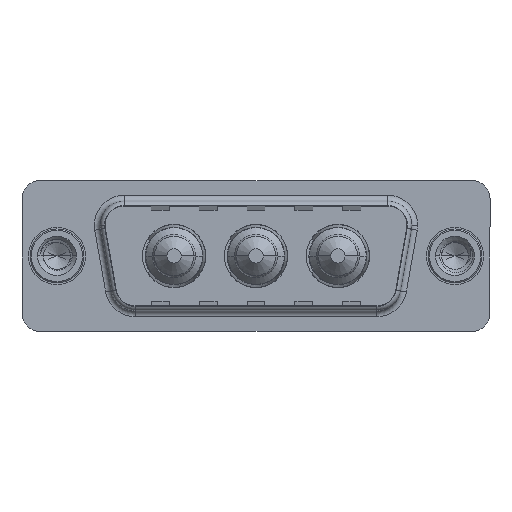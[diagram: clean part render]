
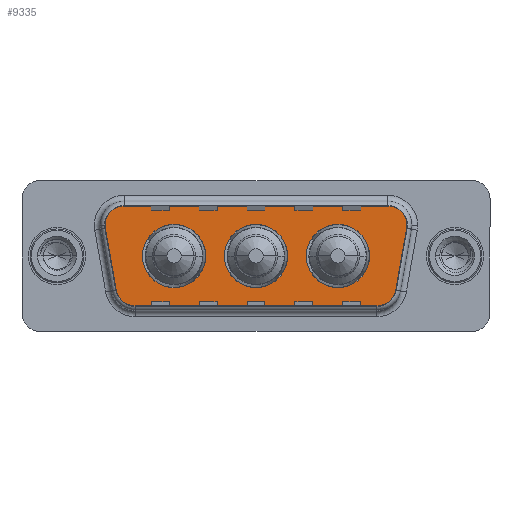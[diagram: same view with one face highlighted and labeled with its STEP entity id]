
A CAD part, top view. The second image highlights one B-rep face of the part: STEP entity #9335.
In plain terms, the highlighted planar face has unit normal (0, 0, 1).
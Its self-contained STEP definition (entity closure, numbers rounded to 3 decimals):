
#252 = CARTESIAN_POINT ( 'NONE',  ( 5.411, 4.9, 0. ) ) ;
#333 = DIRECTION ( 'NONE',  ( -1., 0., 0. ) ) ;
#359 = FACE_BOUND ( 'NONE', #11732, .T. ) ;
#482 = CARTESIAN_POINT ( 'NONE',  ( 14., 0., 0. ) ) ;
#794 = CARTESIAN_POINT ( 'NONE',  ( 29.859, 2.553, 0. ) ) ;
#1148 = VECTOR ( 'NONE', #8163, 1000. ) ;
#1615 = CIRCLE ( 'NONE', #15062, 2.65 ) ;
#1668 = EDGE_LOOP ( 'NONE', ( #4404, #13448 ) ) ;
#1833 = AXIS2_PLACEMENT_3D ( 'NONE', #14568, #5137, #16014 ) ;
#2501 = DIRECTION ( 'NONE',  ( 1., 0., 0. ) ) ;
#2558 = CARTESIAN_POINT ( 'NONE',  ( 16.65, 0., 0. ) ) ;
#2689 = DIRECTION ( 'NONE',  ( 0., 0., 1. ) ) ;
#2873 = VERTEX_POINT ( 'NONE', #482 ) ;
#3039 = CARTESIAN_POINT ( 'NONE',  ( 6.434, -4.9, 0. ) ) ;
#3252 = CARTESIAN_POINT ( 'NONE',  ( 12.45, 0., 0. ) ) ;
#3286 = VERTEX_POINT ( 'NONE', #19120 ) ;
#3309 = EDGE_CURVE ( 'NONE', #6683, #13294, #7062, .T. ) ;
#3829 = AXIS2_PLACEMENT_3D ( 'NONE', #7173, #17907, #8789 ) ;
#3975 = FACE_BOUND ( 'NONE', #1668, .T. ) ;
#3980 = CARTESIAN_POINT ( 'NONE',  ( 26.866, -2.9, 0. ) ) ;
#4006 = CARTESIAN_POINT ( 'NONE',  ( 6.434, -4.9, 0. ) ) ;
#4015 = DIRECTION ( 'NONE',  ( 0., 0., 1. ) ) ;
#4022 = CARTESIAN_POINT ( 'NONE',  ( 27.889, 2.9, 0. ) ) ;
#4078 = EDGE_CURVE ( 'NONE', #5817, #15979, #13440, .T. ) ;
#4096 = DIRECTION ( 'NONE',  ( 1., 0., 0. ) ) ;
#4179 = VERTEX_POINT ( 'NONE', #252 ) ;
#4404 = ORIENTED_EDGE ( 'NONE', *, *, #16567, .F. ) ;
#4530 = ORIENTED_EDGE ( 'NONE', *, *, #15115, .T. ) ;
#4539 = CARTESIAN_POINT ( 'NONE',  ( 7.15, 0., 0. ) ) ;
#4577 = CARTESIAN_POINT ( 'NONE',  ( 9.8, 0., 0. ) ) ;
#4589 = DIRECTION ( 'NONE',  ( 0., 0., 1. ) ) ;
#4745 = VECTOR ( 'NONE', #19899, 1000. ) ;
#4818 = VERTEX_POINT ( 'NONE', #15061 ) ;
#4990 = CARTESIAN_POINT ( 'NONE',  ( 5.411, 2.9, 0. ) ) ;
#5137 = DIRECTION ( 'NONE',  ( 0., 0., 1. ) ) ;
#5651 = ORIENTED_EDGE ( 'NONE', *, *, #4078, .F. ) ;
#5777 = LINE ( 'NONE', #11370, #1148 ) ;
#5817 = VERTEX_POINT ( 'NONE', #3252 ) ;
#5860 = AXIS2_PLACEMENT_3D ( 'NONE', #3980, #11973, #2501 ) ;
#5919 = EDGE_CURVE ( 'NONE', #16298, #8431, #14353, .T. ) ;
#6026 = VECTOR ( 'NONE', #16342, 1000. ) ;
#6195 = DIRECTION ( 'NONE',  ( 1., 0., 0. ) ) ;
#6215 = EDGE_CURVE ( 'NONE', #19218, #4818, #6723, .T. ) ;
#6226 = CARTESIAN_POINT ( 'NONE',  ( 26.15, 0., 0. ) ) ;
#6251 = CARTESIAN_POINT ( 'NONE',  ( 23.5, 0., 0. ) ) ;
#6263 = VERTEX_POINT ( 'NONE', #17975 ) ;
#6264 = EDGE_CURVE ( 'NONE', #2873, #7262, #17558, .T. ) ;
#6441 = DIRECTION ( 'NONE',  ( 1., 0., 0. ) ) ;
#6628 = DIRECTION ( 'NONE',  ( 1., 0., 0. ) ) ;
#6683 = VERTEX_POINT ( 'NONE', #19799 ) ;
#6723 = CIRCLE ( 'NONE', #3829, 2.65 ) ;
#6942 = DIRECTION ( 'NONE',  ( 0., 0., 1. ) ) ;
#6947 = CARTESIAN_POINT ( 'NONE',  ( 9.8, 0., 0. ) ) ;
#7012 = DIRECTION ( 'NONE',  ( 0.174, 0.985, 0. ) ) ;
#7062 = CIRCLE ( 'NONE', #19396, 2. ) ;
#7173 = CARTESIAN_POINT ( 'NONE',  ( 23.5, 0., 0. ) ) ;
#7262 = VERTEX_POINT ( 'NONE', #16443 ) ;
#7380 = CARTESIAN_POINT ( 'NONE',  ( 29.859, 2.553, 0. ) ) ;
#7455 = EDGE_CURVE ( 'NONE', #15979, #5817, #15241, .T. ) ;
#7823 = VERTEX_POINT ( 'NONE', #18087 ) ;
#7849 = DIRECTION ( 'NONE',  ( 1., 0., 0. ) ) ;
#7920 = AXIS2_PLACEMENT_3D ( 'NONE', #12153, #2689, #13696 ) ;
#8163 = DIRECTION ( 'NONE',  ( -1., 0., 0. ) ) ;
#8219 = FACE_BOUND ( 'NONE', #15372, .T. ) ;
#8285 = ORIENTED_EDGE ( 'NONE', *, *, #14871, .T. ) ;
#8373 = ORIENTED_EDGE ( 'NONE', *, *, #6215, .F. ) ;
#8431 = VERTEX_POINT ( 'NONE', #4006 ) ;
#8505 = AXIS2_PLACEMENT_3D ( 'NONE', #18816, #9777, #333 ) ;
#8544 = CIRCLE ( 'NONE', #1833, 2. ) ;
#8555 = ORIENTED_EDGE ( 'NONE', *, *, #10106, .T. ) ;
#8789 = DIRECTION ( 'NONE',  ( 1., 0., 0. ) ) ;
#8820 = ORIENTED_EDGE ( 'NONE', *, *, #7455, .F. ) ;
#9335 = ADVANCED_FACE ( 'NONE', ( #3975, #8219, #359, #19832 ), #10388, .T. ) ;
#9551 = ORIENTED_EDGE ( 'NONE', *, *, #17313, .T. ) ;
#9777 = DIRECTION ( 'NONE',  ( 0., 0., 1. ) ) ;
#9946 = VECTOR ( 'NONE', #7012, 1000. ) ;
#9954 = AXIS2_PLACEMENT_3D ( 'NONE', #4990, #15885, #6628 ) ;
#10106 = EDGE_CURVE ( 'NONE', #3286, #19796, #14539, .T. ) ;
#10279 = LINE ( 'NONE', #14810, #6026 ) ;
#10388 = PLANE ( 'NONE',  #5860 ) ;
#10881 = AXIS2_PLACEMENT_3D ( 'NONE', #14055, #4589, #15518 ) ;
#11247 = CIRCLE ( 'NONE', #9954, 2. ) ;
#11281 = AXIS2_PLACEMENT_3D ( 'NONE', #6947, #6942, #6441 ) ;
#11370 = CARTESIAN_POINT ( 'NONE',  ( 5.411, 4.9, 0. ) ) ;
#11732 = EDGE_LOOP ( 'NONE', ( #5651, #8820 ) ) ;
#11973 = DIRECTION ( 'NONE',  ( 0., 0., 1. ) ) ;
#12153 = CARTESIAN_POINT ( 'NONE',  ( 16.65, 0., 0. ) ) ;
#12320 = AXIS2_PLACEMENT_3D ( 'NONE', #2558, #13556, #4096 ) ;
#12523 = EDGE_LOOP ( 'NONE', ( #14360, #8555, #16471, #17594, #8285, #17183, #4530, #17198, #9551 ) ) ;
#12856 = AXIS2_PLACEMENT_3D ( 'NONE', #4577, #15508, #6195 ) ;
#13294 = VERTEX_POINT ( 'NONE', #15830 ) ;
#13440 = CIRCLE ( 'NONE', #11281, 2.65 ) ;
#13448 = ORIENTED_EDGE ( 'NONE', *, *, #6264, .F. ) ;
#13556 = DIRECTION ( 'NONE',  ( 0., 0., 1. ) ) ;
#13696 = DIRECTION ( 'NONE',  ( 1., 0., 0. ) ) ;
#14055 = CARTESIAN_POINT ( 'NONE',  ( 27.889, 2.9, 0. ) ) ;
#14353 = CIRCLE ( 'NONE', #8505, 2. ) ;
#14360 = ORIENTED_EDGE ( 'NONE', *, *, #14970, .T. ) ;
#14539 = LINE ( 'NONE', #794, #9946 ) ;
#14568 = CARTESIAN_POINT ( 'NONE',  ( 26.866, -2.9, 0. ) ) ;
#14810 = CARTESIAN_POINT ( 'NONE',  ( 3.441, 2.553, 0. ) ) ;
#14871 = EDGE_CURVE ( 'NONE', #13294, #4179, #5777, .T. ) ;
#14970 = EDGE_CURVE ( 'NONE', #6263, #3286, #8544, .T. ) ;
#15061 = CARTESIAN_POINT ( 'NONE',  ( 20.85, 0., 0. ) ) ;
#15062 = AXIS2_PLACEMENT_3D ( 'NONE', #6251, #17036, #7849 ) ;
#15115 = EDGE_CURVE ( 'NONE', #7823, #16298, #10279, .T. ) ;
#15241 = CIRCLE ( 'NONE', #12856, 2.65 ) ;
#15340 = ORIENTED_EDGE ( 'NONE', *, *, #15415, .F. ) ;
#15372 = EDGE_LOOP ( 'NONE', ( #8373, #15340 ) ) ;
#15415 = EDGE_CURVE ( 'NONE', #4818, #19218, #1615, .T. ) ;
#15478 = CIRCLE ( 'NONE', #7920, 2.65 ) ;
#15508 = DIRECTION ( 'NONE',  ( 0., 0., 1. ) ) ;
#15518 = DIRECTION ( 'NONE',  ( -1., 0., 0. ) ) ;
#15830 = CARTESIAN_POINT ( 'NONE',  ( 27.889, 4.9, 0. ) ) ;
#15885 = DIRECTION ( 'NONE',  ( 0., 0., 1. ) ) ;
#15979 = VERTEX_POINT ( 'NONE', #4539 ) ;
#16014 = DIRECTION ( 'NONE',  ( 1., 0., 0. ) ) ;
#16298 = VERTEX_POINT ( 'NONE', #17613 ) ;
#16342 = DIRECTION ( 'NONE',  ( 0.174, -0.985, 0. ) ) ;
#16443 = CARTESIAN_POINT ( 'NONE',  ( 19.3, 0., 0. ) ) ;
#16471 = ORIENTED_EDGE ( 'NONE', *, *, #18320, .T. ) ;
#16567 = EDGE_CURVE ( 'NONE', #7262, #2873, #15478, .T. ) ;
#17036 = DIRECTION ( 'NONE',  ( 0., 0., 1. ) ) ;
#17043 = DIRECTION ( 'NONE',  ( -1., 0., 0. ) ) ;
#17183 = ORIENTED_EDGE ( 'NONE', *, *, #17468, .T. ) ;
#17198 = ORIENTED_EDGE ( 'NONE', *, *, #5919, .T. ) ;
#17313 = EDGE_CURVE ( 'NONE', #8431, #6263, #17600, .T. ) ;
#17468 = EDGE_CURVE ( 'NONE', #4179, #7823, #11247, .T. ) ;
#17558 = CIRCLE ( 'NONE', #12320, 2.65 ) ;
#17594 = ORIENTED_EDGE ( 'NONE', *, *, #3309, .T. ) ;
#17600 = LINE ( 'NONE', #3039, #4745 ) ;
#17613 = CARTESIAN_POINT ( 'NONE',  ( 4.464, -3.247, 0. ) ) ;
#17907 = DIRECTION ( 'NONE',  ( 0., 0., 1. ) ) ;
#17975 = CARTESIAN_POINT ( 'NONE',  ( 26.866, -4.9, 0. ) ) ;
#18087 = CARTESIAN_POINT ( 'NONE',  ( 3.441, 2.553, 0. ) ) ;
#18320 = EDGE_CURVE ( 'NONE', #19796, #6683, #18942, .T. ) ;
#18816 = CARTESIAN_POINT ( 'NONE',  ( 6.434, -2.9, 0. ) ) ;
#18942 = CIRCLE ( 'NONE', #10881, 2. ) ;
#19120 = CARTESIAN_POINT ( 'NONE',  ( 28.836, -3.247, 0. ) ) ;
#19218 = VERTEX_POINT ( 'NONE', #6226 ) ;
#19396 = AXIS2_PLACEMENT_3D ( 'NONE', #4022, #4015, #17043 ) ;
#19796 = VERTEX_POINT ( 'NONE', #7380 ) ;
#19799 = CARTESIAN_POINT ( 'NONE',  ( 29.889, 2.9, 0. ) ) ;
#19832 = FACE_OUTER_BOUND ( 'NONE', #12523, .T. ) ;
#19899 = DIRECTION ( 'NONE',  ( 1., 0., 0. ) ) ;
